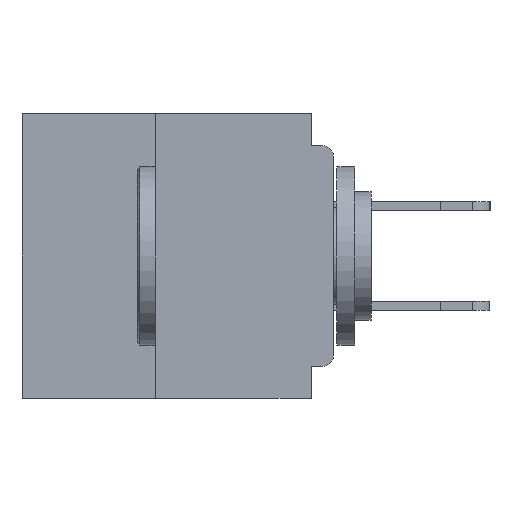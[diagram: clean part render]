
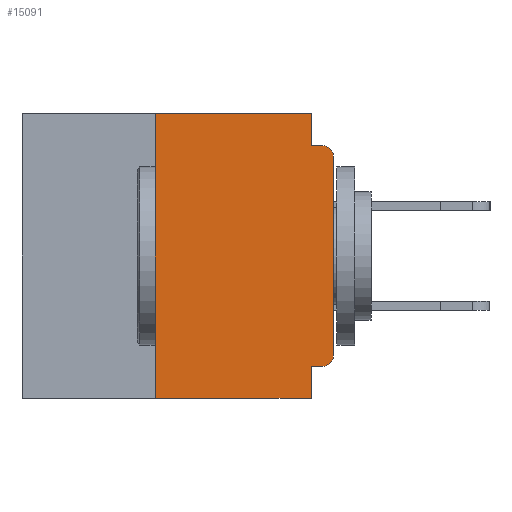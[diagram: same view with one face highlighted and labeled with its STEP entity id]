
A CAD part, left-side view. The second image highlights one B-rep face of the part: STEP entity #15091.
In plain terms, the highlighted planar face has unit normal (-1, 0, 0).
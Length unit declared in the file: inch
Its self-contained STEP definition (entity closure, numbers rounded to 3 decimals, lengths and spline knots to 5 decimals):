
#117 = VECTOR ( 'NONE', #6721, 39.37008 ) ;
#705 = LINE ( 'NONE', #8698, #15709 ) ;
#741 = LINE ( 'NONE', #33201, #6858 ) ;
#1019 = VERTEX_POINT ( 'NONE', #17736 ) ;
#1126 = VERTEX_POINT ( 'NONE', #6350 ) ;
#2414 = ORIENTED_EDGE ( 'NONE', *, *, #35347, .F. ) ;
#2762 = VERTEX_POINT ( 'NONE', #36677 ) ;
#3292 = VECTOR ( 'NONE', #25788, 39.37008 ) ;
#3455 = DIRECTION ( 'NONE',  ( 0., 0., -1. ) ) ;
#3538 = DIRECTION ( 'NONE',  ( -1., 0., 0. ) ) ;
#3589 = CARTESIAN_POINT ( 'NONE',  ( 0., 0.015, -0.06 ) ) ;
#3716 = CARTESIAN_POINT ( 'NONE',  ( 0., 0.437, 0. ) ) ;
#5313 = DIRECTION ( 'NONE',  ( 0., 0., -1. ) ) ;
#6350 = CARTESIAN_POINT ( 'NONE',  ( 0., 0.25, -0.4 ) ) ;
#6485 = EDGE_CURVE ( 'NONE', #13372, #28907, #24299, .T. ) ;
#6721 = DIRECTION ( 'NONE',  ( 0., -1., 0. ) ) ;
#6858 = VECTOR ( 'NONE', #12868, 39.37008 ) ;
#7248 = EDGE_CURVE ( 'NONE', #2762, #28907, #7735, .T. ) ;
#7735 = CIRCLE ( 'NONE', #26751, 0.015 ) ;
#8308 = LINE ( 'NONE', #32306, #23061 ) ;
#8698 = CARTESIAN_POINT ( 'NONE',  ( 0., 0.031, 0. ) ) ;
#9630 = VERTEX_POINT ( 'NONE', #20790 ) ;
#10046 = VERTEX_POINT ( 'NONE', #14067 ) ;
#10082 = EDGE_CURVE ( 'NONE', #37331, #9630, #33809, .T. ) ;
#11004 = ORIENTED_EDGE ( 'NONE', *, *, #24864, .F. ) ;
#11087 = CARTESIAN_POINT ( 'NONE',  ( 0., 0.031, 0. ) ) ;
#11279 = CARTESIAN_POINT ( 'NONE',  ( 0., 0.015, -0.34 ) ) ;
#11677 = DIRECTION ( 'NONE',  ( 0., 0., -1. ) ) ;
#12371 = ORIENTED_EDGE ( 'NONE', *, *, #31899, .F. ) ;
#12795 = ORIENTED_EDGE ( 'NONE', *, *, #36827, .F. ) ;
#12868 = DIRECTION ( 'NONE',  ( 0., -1., 0. ) ) ;
#12960 = CARTESIAN_POINT ( 'NONE',  ( 0., 0.015, -0.045 ) ) ;
#13372 = VERTEX_POINT ( 'NONE', #17961 ) ;
#14067 = CARTESIAN_POINT ( 'NONE',  ( 0., 0.25, 0. ) ) ;
#14289 = CARTESIAN_POINT ( 'NONE',  ( 0., 0.437, 0. ) ) ;
#14295 = DIRECTION ( 'NONE',  ( 0., 0., -1. ) ) ;
#15091 = ADVANCED_FACE ( 'NONE', ( #29018 ), #25877, .F. ) ;
#15709 = VECTOR ( 'NONE', #11677, 39.37008 ) ;
#16048 = LINE ( 'NONE', #3716, #117 ) ;
#16581 = VECTOR ( 'NONE', #18509, 39.37008 ) ;
#17260 = DIRECTION ( 'NONE',  ( 0., 0., -1. ) ) ;
#17736 = CARTESIAN_POINT ( 'NONE',  ( 0., 0.015, -0.355 ) ) ;
#17870 = VECTOR ( 'NONE', #32840, 39.37008 ) ;
#17913 = DIRECTION ( 'NONE',  ( 0., 0., 1. ) ) ;
#17961 = CARTESIAN_POINT ( 'NONE',  ( 0., 0.031, -0.045 ) ) ;
#18283 = EDGE_CURVE ( 'NONE', #1019, #21760, #36067, .T. ) ;
#18433 = EDGE_CURVE ( 'NONE', #21760, #2762, #8308, .T. ) ;
#18509 = DIRECTION ( 'NONE',  ( 0., -1., 0. ) ) ;
#18662 = CARTESIAN_POINT ( 'NONE',  ( 0., 0., -0.045 ) ) ;
#20052 = LINE ( 'NONE', #22885, #3292 ) ;
#20119 = CARTESIAN_POINT ( 'NONE',  ( 0., 0.031, -0.4 ) ) ;
#20608 = ORIENTED_EDGE ( 'NONE', *, *, #34982, .T. ) ;
#20790 = CARTESIAN_POINT ( 'NONE',  ( 0., 0.031, -0.4 ) ) ;
#20917 = AXIS2_PLACEMENT_3D ( 'NONE', #11279, #31689, #14295 ) ;
#21760 = VERTEX_POINT ( 'NONE', #27495 ) ;
#22396 = ORIENTED_EDGE ( 'NONE', *, *, #6485, .F. ) ;
#22885 = CARTESIAN_POINT ( 'NONE',  ( 0., 0., -0.355 ) ) ;
#23061 = VECTOR ( 'NONE', #17913, 39.37008 ) ;
#24246 = CARTESIAN_POINT ( 'NONE',  ( 0., 0.25, -0.4 ) ) ;
#24299 = LINE ( 'NONE', #18662, #16581 ) ;
#24864 = EDGE_CURVE ( 'NONE', #10046, #33126, #16048, .T. ) ;
#25788 = DIRECTION ( 'NONE',  ( 0., 1., 0. ) ) ;
#25877 = PLANE ( 'NONE',  #32691 ) ;
#26443 = LINE ( 'NONE', #24246, #17870 ) ;
#26751 = AXIS2_PLACEMENT_3D ( 'NONE', #3589, #3538, #3455 ) ;
#27420 = ORIENTED_EDGE ( 'NONE', *, *, #10082, .F. ) ;
#27495 = CARTESIAN_POINT ( 'NONE',  ( 0., 0., -0.34 ) ) ;
#28834 = ORIENTED_EDGE ( 'NONE', *, *, #7248, .T. ) ;
#28907 = VERTEX_POINT ( 'NONE', #12960 ) ;
#29018 = FACE_OUTER_BOUND ( 'NONE', #36417, .T. ) ;
#31689 = DIRECTION ( 'NONE',  ( -1., 0., 0. ) ) ;
#31899 = EDGE_CURVE ( 'NONE', #1019, #37331, #20052, .T. ) ;
#32306 = CARTESIAN_POINT ( 'NONE',  ( 0., 0., 0. ) ) ;
#32691 = AXIS2_PLACEMENT_3D ( 'NONE', #14289, #34531, #17260 ) ;
#32840 = DIRECTION ( 'NONE',  ( 0., 0., 1. ) ) ;
#32952 = ORIENTED_EDGE ( 'NONE', *, *, #18433, .T. ) ;
#33126 = VERTEX_POINT ( 'NONE', #11087 ) ;
#33201 = CARTESIAN_POINT ( 'NONE',  ( 0., 0.437, -0.4 ) ) ;
#33809 = LINE ( 'NONE', #20119, #34694 ) ;
#34531 = DIRECTION ( 'NONE',  ( 1., 0., 0. ) ) ;
#34694 = VECTOR ( 'NONE', #5313, 39.37008 ) ;
#34982 = EDGE_CURVE ( 'NONE', #1126, #9630, #741, .T. ) ;
#35347 = EDGE_CURVE ( 'NONE', #33126, #13372, #705, .T. ) ;
#35632 = CARTESIAN_POINT ( 'NONE',  ( 0., 0.031, -0.355 ) ) ;
#36067 = CIRCLE ( 'NONE', #20917, 0.015 ) ;
#36417 = EDGE_LOOP ( 'NONE', ( #32952, #28834, #22396, #2414, #11004, #12795, #20608, #27420, #12371, #37261 ) ) ;
#36677 = CARTESIAN_POINT ( 'NONE',  ( 0., 0., -0.06 ) ) ;
#36827 = EDGE_CURVE ( 'NONE', #1126, #10046, #26443, .T. ) ;
#37261 = ORIENTED_EDGE ( 'NONE', *, *, #18283, .T. ) ;
#37331 = VERTEX_POINT ( 'NONE', #35632 ) ;
